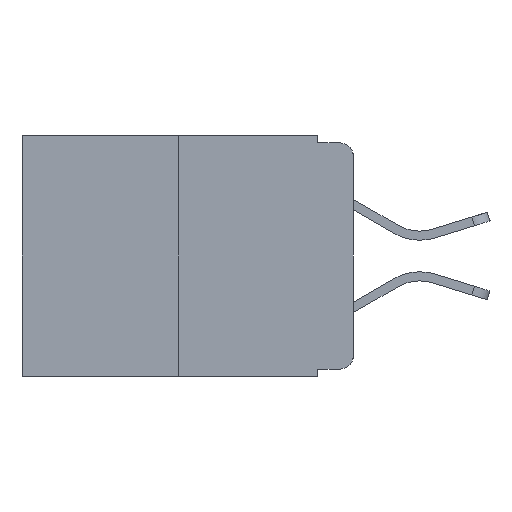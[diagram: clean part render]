
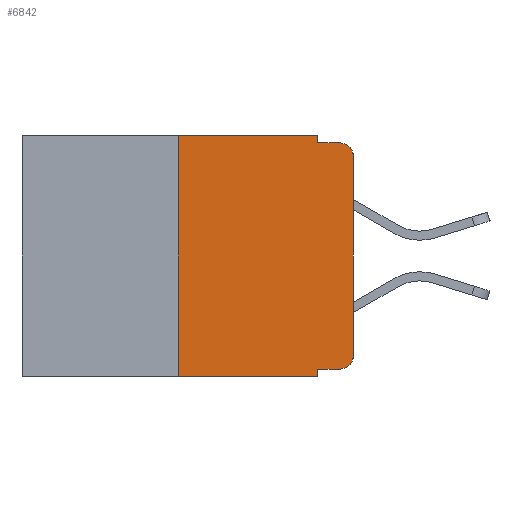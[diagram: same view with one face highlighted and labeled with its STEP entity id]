
A CAD part, left-side view. The second image highlights one B-rep face of the part: STEP entity #6842.
In plain terms, the highlighted planar face has unit normal (-1, 0, 0).
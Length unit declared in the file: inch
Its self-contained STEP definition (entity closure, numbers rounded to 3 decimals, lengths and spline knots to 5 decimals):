
#303 = VECTOR ( 'NONE', #1264, 39.37008 ) ;
#914 = VECTOR ( 'NONE', #13684, 39.37008 ) ;
#1264 = DIRECTION ( 'NONE',  ( 0., -1., 0. ) ) ;
#1271 = LINE ( 'NONE', #23599, #16006 ) ;
#1375 = VECTOR ( 'NONE', #12432, 39.37008 ) ;
#1533 = EDGE_CURVE ( 'NONE', #5965, #6162, #11073, .T. ) ;
#2026 = CARTESIAN_POINT ( 'NONE',  ( 0., 0.02, -0.333 ) ) ;
#2203 = LINE ( 'NONE', #17403, #914 ) ;
#2487 = AXIS2_PLACEMENT_3D ( 'NONE', #4914, #18275, #6828 ) ;
#3033 = CARTESIAN_POINT ( 'NONE',  ( 0., 0.473, -0.343 ) ) ;
#3051 = ORIENTED_EDGE ( 'NONE', *, *, #1533, .T. ) ;
#3107 = CIRCLE ( 'NONE', #22430, 0.02 ) ;
#3222 = VERTEX_POINT ( 'NONE', #7073 ) ;
#3333 = LINE ( 'NONE', #4044, #19156 ) ;
#3588 = PLANE ( 'NONE',  #16178 ) ;
#3625 = CARTESIAN_POINT ( 'NONE',  ( 0., 0.051, -0.333 ) ) ;
#4041 = DIRECTION ( 'NONE',  ( -1., 0., 0. ) ) ;
#4044 = CARTESIAN_POINT ( 'NONE',  ( 0., 0.25, 0. ) ) ;
#4733 = DIRECTION ( 'NONE',  ( 0., 0., -1. ) ) ;
#4914 = CARTESIAN_POINT ( 'NONE',  ( 0., 0.02, -0.313 ) ) ;
#4962 = LINE ( 'NONE', #6630, #24551 ) ;
#4979 = DIRECTION ( 'NONE',  ( 0., -1., 0. ) ) ;
#5964 = VERTEX_POINT ( 'NONE', #2026 ) ;
#5965 = VERTEX_POINT ( 'NONE', #24723 ) ;
#6162 = VERTEX_POINT ( 'NONE', #19022 ) ;
#6630 = CARTESIAN_POINT ( 'NONE',  ( 0., 0.051, 0. ) ) ;
#6828 = DIRECTION ( 'NONE',  ( 0., 0., -1. ) ) ;
#6842 = ADVANCED_FACE ( 'NONE', ( #11268 ), #3588, .F. ) ;
#7003 = VERTEX_POINT ( 'NONE', #9106 ) ;
#7073 = CARTESIAN_POINT ( 'NONE',  ( 0., 0.051, 0. ) ) ;
#7200 = ORIENTED_EDGE ( 'NONE', *, *, #7231, .F. ) ;
#7231 = EDGE_CURVE ( 'NONE', #7003, #3222, #2203, .T. ) ;
#7311 = CARTESIAN_POINT ( 'NONE',  ( 0., 0.051, -0.01 ) ) ;
#7815 = EDGE_CURVE ( 'NONE', #6162, #12136, #3107, .T. ) ;
#8734 = DIRECTION ( 'NONE',  ( 0., 0., -1. ) ) ;
#9106 = CARTESIAN_POINT ( 'NONE',  ( 0., 0.25, 0. ) ) ;
#9268 = ORIENTED_EDGE ( 'NONE', *, *, #21443, .T. ) ;
#9668 = EDGE_CURVE ( 'NONE', #11376, #7003, #3333, .T. ) ;
#10119 = CIRCLE ( 'NONE', #2487, 0.02 ) ;
#10478 = DIRECTION ( 'NONE',  ( 0., 0., -1. ) ) ;
#10668 = EDGE_CURVE ( 'NONE', #3222, #13248, #16710, .T. ) ;
#10766 = DIRECTION ( 'NONE',  ( 1., 0., 0. ) ) ;
#10803 = CARTESIAN_POINT ( 'NONE',  ( 0., 0.473, 0. ) ) ;
#11073 = LINE ( 'NONE', #17653, #1375 ) ;
#11268 = FACE_OUTER_BOUND ( 'NONE', #19313, .T. ) ;
#11376 = VERTEX_POINT ( 'NONE', #16428 ) ;
#12135 = CARTESIAN_POINT ( 'NONE',  ( 0., 0.051, -0.343 ) ) ;
#12136 = VERTEX_POINT ( 'NONE', #12387 ) ;
#12219 = EDGE_CURVE ( 'NONE', #5964, #5965, #10119, .T. ) ;
#12387 = CARTESIAN_POINT ( 'NONE',  ( 0., 0.02, -0.01 ) ) ;
#12389 = ORIENTED_EDGE ( 'NONE', *, *, #17120, .T. ) ;
#12432 = DIRECTION ( 'NONE',  ( 0., 0., 1. ) ) ;
#12474 = LINE ( 'NONE', #3033, #21981 ) ;
#13001 = ORIENTED_EDGE ( 'NONE', *, *, #24139, .F. ) ;
#13248 = VERTEX_POINT ( 'NONE', #7311 ) ;
#13579 = ORIENTED_EDGE ( 'NONE', *, *, #12219, .T. ) ;
#13684 = DIRECTION ( 'NONE',  ( 0., -1., 0. ) ) ;
#14168 = DIRECTION ( 'NONE',  ( 0., -1., 0. ) ) ;
#15457 = CARTESIAN_POINT ( 'NONE',  ( 0., 0.02, -0.03 ) ) ;
#15765 = ORIENTED_EDGE ( 'NONE', *, *, #10668, .F. ) ;
#16006 = VECTOR ( 'NONE', #14168, 39.37008 ) ;
#16040 = ORIENTED_EDGE ( 'NONE', *, *, #21508, .F. ) ;
#16178 = AXIS2_PLACEMENT_3D ( 'NONE', #10803, #10766, #10478 ) ;
#16428 = CARTESIAN_POINT ( 'NONE',  ( 0., 0.25, -0.343 ) ) ;
#16552 = VERTEX_POINT ( 'NONE', #12135 ) ;
#16710 = LINE ( 'NONE', #20162, #20622 ) ;
#17120 = EDGE_CURVE ( 'NONE', #22808, #5964, #1271, .T. ) ;
#17369 = DIRECTION ( 'NONE',  ( 0., 0., -1. ) ) ;
#17373 = DIRECTION ( 'NONE',  ( 0., 0., 1. ) ) ;
#17403 = CARTESIAN_POINT ( 'NONE',  ( 0., 0.473, 0. ) ) ;
#17653 = CARTESIAN_POINT ( 'NONE',  ( 0., 0., 0. ) ) ;
#18275 = DIRECTION ( 'NONE',  ( -1., 0., 0. ) ) ;
#19022 = CARTESIAN_POINT ( 'NONE',  ( 0., 0., -0.03 ) ) ;
#19156 = VECTOR ( 'NONE', #17373, 39.37008 ) ;
#19313 = EDGE_LOOP ( 'NONE', ( #3051, #23609, #16040, #15765, #7200, #20636, #9268, #13001, #12389, #13579 ) ) ;
#20162 = CARTESIAN_POINT ( 'NONE',  ( 0., 0.051, 0. ) ) ;
#20622 = VECTOR ( 'NONE', #8734, 39.37008 ) ;
#20636 = ORIENTED_EDGE ( 'NONE', *, *, #9668, .F. ) ;
#20794 = LINE ( 'NONE', #22232, #303 ) ;
#21443 = EDGE_CURVE ( 'NONE', #11376, #16552, #12474, .T. ) ;
#21508 = EDGE_CURVE ( 'NONE', #13248, #12136, #20794, .T. ) ;
#21981 = VECTOR ( 'NONE', #4979, 39.37008 ) ;
#22232 = CARTESIAN_POINT ( 'NONE',  ( 0., 0.051, -0.01 ) ) ;
#22430 = AXIS2_PLACEMENT_3D ( 'NONE', #15457, #4041, #17369 ) ;
#22808 = VERTEX_POINT ( 'NONE', #3625 ) ;
#23599 = CARTESIAN_POINT ( 'NONE',  ( 0., 0.051, -0.333 ) ) ;
#23609 = ORIENTED_EDGE ( 'NONE', *, *, #7815, .T. ) ;
#24139 = EDGE_CURVE ( 'NONE', #22808, #16552, #4962, .T. ) ;
#24551 = VECTOR ( 'NONE', #4733, 39.37008 ) ;
#24723 = CARTESIAN_POINT ( 'NONE',  ( 0., 0., -0.313 ) ) ;
